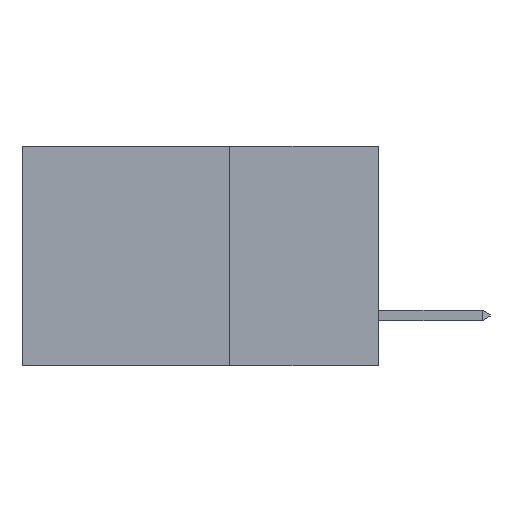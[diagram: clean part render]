
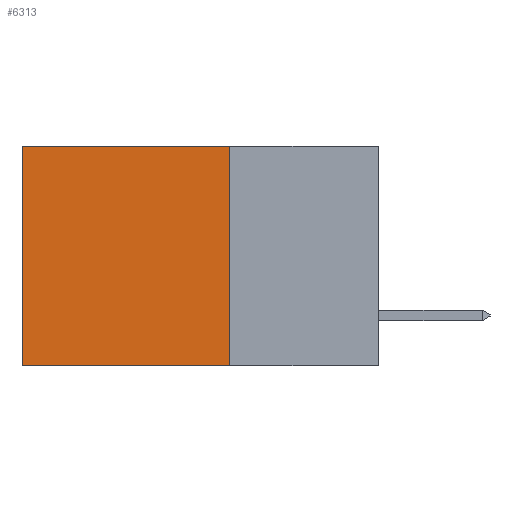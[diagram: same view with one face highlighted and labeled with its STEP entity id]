
A CAD part, left-side view. The second image highlights one B-rep face of the part: STEP entity #6313.
In plain terms, the highlighted planar face has unit normal (-1, 0, 0).
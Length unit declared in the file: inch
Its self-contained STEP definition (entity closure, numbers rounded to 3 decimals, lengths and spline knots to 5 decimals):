
#210 = CARTESIAN_POINT ( 'NONE',  ( 0.298, 0.25, 0. ) ) ;
#227 = VECTOR ( 'NONE', #14855, 39.37008 ) ;
#319 = CARTESIAN_POINT ( 'NONE',  ( 0.298, 0.25, 0. ) ) ;
#757 = EDGE_CURVE ( 'NONE', #11392, #12125, #1234, .T. ) ;
#839 = VECTOR ( 'NONE', #13281, 39.37008 ) ;
#1234 = LINE ( 'NONE', #13101, #839 ) ;
#1268 = ORIENTED_EDGE ( 'NONE', *, *, #8916, .T. ) ;
#2085 = VECTOR ( 'NONE', #15448, 39.37008 ) ;
#2962 = FACE_OUTER_BOUND ( 'NONE', #7743, .T. ) ;
#3029 = DIRECTION ( 'NONE',  ( 0., 1., 0. ) ) ;
#3426 = CARTESIAN_POINT ( 'NONE',  ( 0.298, 0.6, -0.37 ) ) ;
#3788 = ORIENTED_EDGE ( 'NONE', *, *, #757, .F. ) ;
#5137 = EDGE_CURVE ( 'NONE', #15939, #13874, #10309, .T. ) ;
#5900 = ORIENTED_EDGE ( 'NONE', *, *, #5137, .T. ) ;
#6313 = ADVANCED_FACE ( 'NONE', ( #2962 ), #15086, .F. ) ;
#6818 = ORIENTED_EDGE ( 'NONE', *, *, #15626, .F. ) ;
#7743 = EDGE_LOOP ( 'NONE', ( #5900, #6818, #3788, #1268 ) ) ;
#8369 = CARTESIAN_POINT ( 'NONE',  ( 0.298, 0.25, -0.37 ) ) ;
#8609 = VECTOR ( 'NONE', #3029, 39.37008 ) ;
#8896 = LINE ( 'NONE', #8369, #2085 ) ;
#8916 = EDGE_CURVE ( 'NONE', #11392, #15939, #12120, .T. ) ;
#9030 = CARTESIAN_POINT ( 'NONE',  ( 0.298, 0.6, 0. ) ) ;
#9393 = CARTESIAN_POINT ( 'NONE',  ( 0.298, 0.25, 0. ) ) ;
#10309 = LINE ( 'NONE', #11954, #227 ) ;
#11392 = VERTEX_POINT ( 'NONE', #210 ) ;
#11954 = CARTESIAN_POINT ( 'NONE',  ( 0.298, 0.6, 0. ) ) ;
#12120 = LINE ( 'NONE', #9393, #8609 ) ;
#12125 = VERTEX_POINT ( 'NONE', #12817 ) ;
#12817 = CARTESIAN_POINT ( 'NONE',  ( 0.298, 0.25, -0.37 ) ) ;
#13101 = CARTESIAN_POINT ( 'NONE',  ( 0.298, 0.25, 0. ) ) ;
#13281 = DIRECTION ( 'NONE',  ( 0., 0., -1. ) ) ;
#13874 = VERTEX_POINT ( 'NONE', #3426 ) ;
#14729 = DIRECTION ( 'NONE',  ( 0., 0., -1. ) ) ;
#14733 = DIRECTION ( 'NONE',  ( 1., 0., 0. ) ) ;
#14855 = DIRECTION ( 'NONE',  ( 0., 0., -1. ) ) ;
#15086 = PLANE ( 'NONE',  #15775 ) ;
#15448 = DIRECTION ( 'NONE',  ( 0., 1., 0. ) ) ;
#15626 = EDGE_CURVE ( 'NONE', #12125, #13874, #8896, .T. ) ;
#15775 = AXIS2_PLACEMENT_3D ( 'NONE', #319, #14733, #14729 ) ;
#15939 = VERTEX_POINT ( 'NONE', #9030 ) ;
